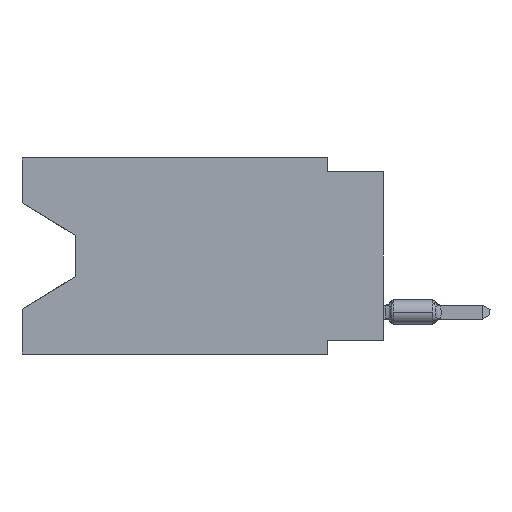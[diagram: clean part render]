
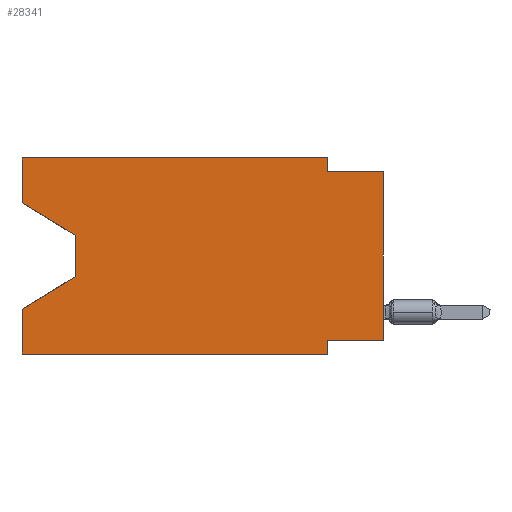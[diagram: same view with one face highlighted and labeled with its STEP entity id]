
A CAD part, left-side view. The second image highlights one B-rep face of the part: STEP entity #28341.
In plain terms, the highlighted planar face has unit normal (-1, 0, 0).
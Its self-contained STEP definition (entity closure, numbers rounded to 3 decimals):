
#113 = LINE ( 'NONE', #8057, #46520 ) ;
#792 = DIRECTION ( 'NONE',  ( 0., 0., -1. ) ) ;
#1389 = DIRECTION ( 'NONE',  ( 0., 0., 1. ) ) ;
#1434 = EDGE_CURVE ( 'NONE', #17182, #42749, #37971, .T. ) ;
#2248 = VERTEX_POINT ( 'NONE', #29635 ) ;
#2362 = EDGE_CURVE ( 'NONE', #2248, #18324, #113, .T. ) ;
#3147 = CARTESIAN_POINT ( 'NONE',  ( 0., 16.383, 0. ) ) ;
#3967 = VECTOR ( 'NONE', #6389, 1000. ) ;
#4549 = ORIENTED_EDGE ( 'NONE', *, *, #41500, .T. ) ;
#6389 = DIRECTION ( 'NONE',  ( 0., 0., -1. ) ) ;
#6634 = ORIENTED_EDGE ( 'NONE', *, *, #30833, .F. ) ;
#6898 = CARTESIAN_POINT ( 'NONE',  ( 0., 16.383, -6.852 ) ) ;
#7192 = ORIENTED_EDGE ( 'NONE', *, *, #15044, .T. ) ;
#7351 = CARTESIAN_POINT ( 'NONE',  ( 0., 2.54, -8.255 ) ) ;
#7463 = CARTESIAN_POINT ( 'NONE',  ( 0., 16.383, 0. ) ) ;
#7665 = DIRECTION ( 'NONE',  ( 0., 0.855, -0.519 ) ) ;
#8057 = CARTESIAN_POINT ( 'NONE',  ( 0., 0., 0. ) ) ;
#9248 = CARTESIAN_POINT ( 'NONE',  ( 0., 2.54, 0. ) ) ;
#9782 = ORIENTED_EDGE ( 'NONE', *, *, #1434, .F. ) ;
#10718 = CARTESIAN_POINT ( 'NONE',  ( 0., 0., -0.635 ) ) ;
#11617 = CARTESIAN_POINT ( 'NONE',  ( 0., 16.383, -8.89 ) ) ;
#11794 = DIRECTION ( 'NONE',  ( 0., -0.855, -0.519 ) ) ;
#11867 = EDGE_CURVE ( 'NONE', #42360, #26866, #13388, .T. ) ;
#12470 = EDGE_CURVE ( 'NONE', #32781, #14269, #15814, .T. ) ;
#12803 = EDGE_CURVE ( 'NONE', #25426, #42360, #33601, .T. ) ;
#13388 = LINE ( 'NONE', #28529, #38789 ) ;
#14269 = VERTEX_POINT ( 'NONE', #24197 ) ;
#14315 = VECTOR ( 'NONE', #32920, 1000. ) ;
#14452 = LINE ( 'NONE', #10718, #29137 ) ;
#14663 = VERTEX_POINT ( 'NONE', #9248 ) ;
#15044 = EDGE_CURVE ( 'NONE', #42458, #42749, #21006, .T. ) ;
#15321 = EDGE_CURVE ( 'NONE', #14269, #14663, #37154, .T. ) ;
#15814 = LINE ( 'NONE', #46795, #48319 ) ;
#15837 = LINE ( 'NONE', #31433, #34680 ) ;
#16490 = CARTESIAN_POINT ( 'NONE',  ( 0., 16.383, -2.038 ) ) ;
#17182 = VERTEX_POINT ( 'NONE', #7351 ) ;
#17213 = ORIENTED_EDGE ( 'NONE', *, *, #41112, .F. ) ;
#18144 = VECTOR ( 'NONE', #45639, 1000. ) ;
#18324 = VERTEX_POINT ( 'NONE', #38072 ) ;
#19366 = ORIENTED_EDGE ( 'NONE', *, *, #15321, .F. ) ;
#19521 = DIRECTION ( 'NONE',  ( 0., -1., 0. ) ) ;
#19810 = FACE_OUTER_BOUND ( 'NONE', #33449, .T. ) ;
#20011 = CARTESIAN_POINT ( 'NONE',  ( 0., 16.383, -2.038 ) ) ;
#20322 = LINE ( 'NONE', #27538, #3967 ) ;
#21006 = LINE ( 'NONE', #44065, #14315 ) ;
#22254 = AXIS2_PLACEMENT_3D ( 'NONE', #42383, #31209, #46352 ) ;
#22594 = DIRECTION ( 'NONE',  ( 0., 0., 1. ) ) ;
#23205 = CARTESIAN_POINT ( 'NONE',  ( 0., 2.54, -0.635 ) ) ;
#23748 = VECTOR ( 'NONE', #22594, 1000. ) ;
#24045 = ORIENTED_EDGE ( 'NONE', *, *, #12803, .T. ) ;
#24197 = CARTESIAN_POINT ( 'NONE',  ( 0., 16.383, 0. ) ) ;
#25426 = VERTEX_POINT ( 'NONE', #32644 ) ;
#25865 = DIRECTION ( 'NONE',  ( 0., -1., 0. ) ) ;
#26484 = ORIENTED_EDGE ( 'NONE', *, *, #11867, .T. ) ;
#26675 = DIRECTION ( 'NONE',  ( 0., 0., 1. ) ) ;
#26753 = ORIENTED_EDGE ( 'NONE', *, *, #46085, .F. ) ;
#26866 = VERTEX_POINT ( 'NONE', #6898 ) ;
#27258 = PLANE ( 'NONE',  #22254 ) ;
#27538 = CARTESIAN_POINT ( 'NONE',  ( 0., 2.54, 0. ) ) ;
#28341 = ADVANCED_FACE ( 'NONE', ( #19810 ), #27258, .F. ) ;
#28529 = CARTESIAN_POINT ( 'NONE',  ( 0., 13.97, -5.385 ) ) ;
#29137 = VECTOR ( 'NONE', #25865, 1000. ) ;
#29360 = VECTOR ( 'NONE', #19521, 1000. ) ;
#29383 = CARTESIAN_POINT ( 'NONE',  ( 0., 13.97, -3.505 ) ) ;
#29635 = CARTESIAN_POINT ( 'NONE',  ( 0., 0., -8.255 ) ) ;
#30511 = CARTESIAN_POINT ( 'NONE',  ( 0., 2.54, -8.89 ) ) ;
#30833 = EDGE_CURVE ( 'NONE', #14663, #39728, #20322, .T. ) ;
#31209 = DIRECTION ( 'NONE',  ( 1., 0., 0. ) ) ;
#31433 = CARTESIAN_POINT ( 'NONE',  ( 0., 0., -8.255 ) ) ;
#32482 = VECTOR ( 'NONE', #792, 1000. ) ;
#32644 = CARTESIAN_POINT ( 'NONE',  ( 0., 13.97, -3.505 ) ) ;
#32781 = VERTEX_POINT ( 'NONE', #20011 ) ;
#32920 = DIRECTION ( 'NONE',  ( 0., -1., 0. ) ) ;
#33449 = EDGE_LOOP ( 'NONE', ( #4549, #24045, #26484, #40143, #7192, #9782, #17213, #34352, #26753, #6634, #19366, #47926 ) ) ;
#33601 = LINE ( 'NONE', #29383, #32482 ) ;
#34352 = ORIENTED_EDGE ( 'NONE', *, *, #2362, .T. ) ;
#34680 = VECTOR ( 'NONE', #46332, 1000. ) ;
#37154 = LINE ( 'NONE', #3147, #29360 ) ;
#37971 = LINE ( 'NONE', #30511, #18144 ) ;
#38072 = CARTESIAN_POINT ( 'NONE',  ( 0., 0., -0.635 ) ) ;
#38789 = VECTOR ( 'NONE', #7665, 1000. ) ;
#39728 = VERTEX_POINT ( 'NONE', #23205 ) ;
#40143 = ORIENTED_EDGE ( 'NONE', *, *, #48856, .F. ) ;
#40193 = VECTOR ( 'NONE', #11794, 1000. ) ;
#41112 = EDGE_CURVE ( 'NONE', #2248, #17182, #15837, .T. ) ;
#41500 = EDGE_CURVE ( 'NONE', #32781, #25426, #46512, .T. ) ;
#42360 = VERTEX_POINT ( 'NONE', #47363 ) ;
#42383 = CARTESIAN_POINT ( 'NONE',  ( 0., 16.383, 0. ) ) ;
#42458 = VERTEX_POINT ( 'NONE', #11617 ) ;
#42749 = VERTEX_POINT ( 'NONE', #45540 ) ;
#44065 = CARTESIAN_POINT ( 'NONE',  ( 0., 16.383, -8.89 ) ) ;
#45540 = CARTESIAN_POINT ( 'NONE',  ( 0., 2.54, -8.89 ) ) ;
#45639 = DIRECTION ( 'NONE',  ( 0., 0., -1. ) ) ;
#46085 = EDGE_CURVE ( 'NONE', #39728, #18324, #14452, .T. ) ;
#46332 = DIRECTION ( 'NONE',  ( 0., 1., 0. ) ) ;
#46352 = DIRECTION ( 'NONE',  ( 0., 0., -1. ) ) ;
#46416 = LINE ( 'NONE', #7463, #23748 ) ;
#46512 = LINE ( 'NONE', #16490, #40193 ) ;
#46520 = VECTOR ( 'NONE', #26675, 1000. ) ;
#46795 = CARTESIAN_POINT ( 'NONE',  ( 0., 16.383, 0. ) ) ;
#47363 = CARTESIAN_POINT ( 'NONE',  ( 0., 13.97, -5.385 ) ) ;
#47926 = ORIENTED_EDGE ( 'NONE', *, *, #12470, .F. ) ;
#48319 = VECTOR ( 'NONE', #1389, 1000. ) ;
#48856 = EDGE_CURVE ( 'NONE', #42458, #26866, #46416, .T. ) ;
